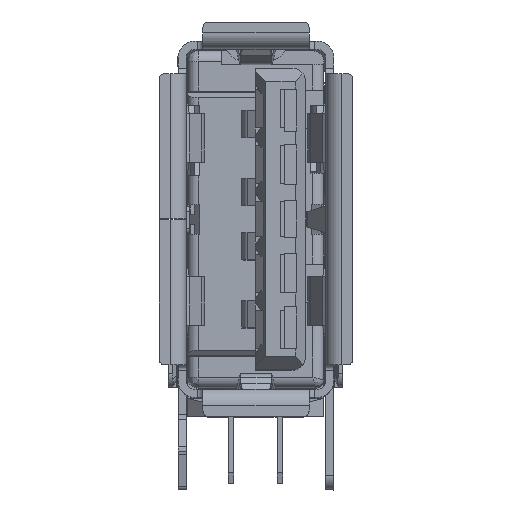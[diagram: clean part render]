
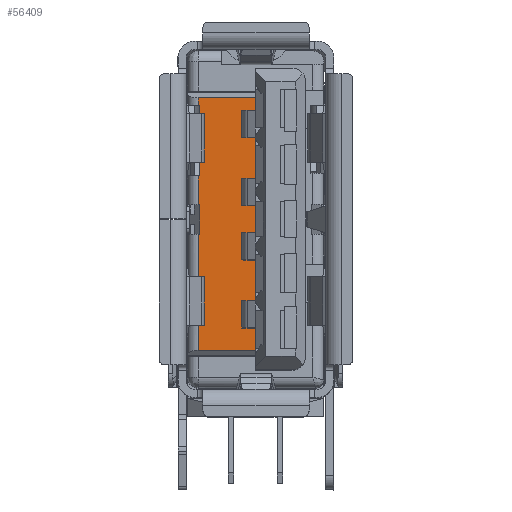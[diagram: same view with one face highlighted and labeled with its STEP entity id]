
A CAD part, top view. The second image highlights one B-rep face of the part: STEP entity #56409.
In plain terms, the highlighted planar face has unit normal (0, 0, 1).
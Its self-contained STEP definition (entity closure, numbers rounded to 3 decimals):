
#46 = ORIENTED_EDGE ( 'NONE', *, *, #74135, .T. ) ;
#1240 = VECTOR ( 'NONE', #19830, 1000. ) ;
#2455 = ORIENTED_EDGE ( 'NONE', *, *, #68808, .T. ) ;
#4025 = VECTOR ( 'NONE', #60709, 1000. ) ;
#4197 = AXIS2_PLACEMENT_3D ( 'NONE', #62936, #84870, #19425 ) ;
#5372 = DIRECTION ( 'NONE',  ( -1., 0., 0. ) ) ;
#6657 = ORIENTED_EDGE ( 'NONE', *, *, #52125, .T. ) ;
#6855 = EDGE_CURVE ( 'NONE', #19934, #87903, #26088, .T. ) ;
#7432 = VECTOR ( 'NONE', #47009, 1000. ) ;
#11514 = VERTEX_POINT ( 'NONE', #66420 ) ;
#12443 = EDGE_CURVE ( 'NONE', #89733, #81826, #86185, .T. ) ;
#12516 = LINE ( 'NONE', #71252, #74132 ) ;
#13197 = FACE_OUTER_BOUND ( 'NONE', #21244, .T. ) ;
#14229 = LINE ( 'NONE', #50551, #50821 ) ;
#14519 = DIRECTION ( 'NONE',  ( -1., 0., 0. ) ) ;
#14822 = ORIENTED_EDGE ( 'NONE', *, *, #34793, .T. ) ;
#16552 = VECTOR ( 'NONE', #48898, 1000. ) ;
#16812 = VERTEX_POINT ( 'NONE', #84341 ) ;
#17603 = DIRECTION ( 'NONE',  ( 1., 0., 0. ) ) ;
#17866 = CARTESIAN_POINT ( 'NONE',  ( -1.055, 0.55, -10.48 ) ) ;
#18363 = EDGE_CURVE ( 'NONE', #81826, #60747, #56077, .T. ) ;
#19425 = DIRECTION ( 'NONE',  ( 0., 1., 0. ) ) ;
#19491 = EDGE_CURVE ( 'NONE', #64188, #16812, #32213, .T. ) ;
#19830 = DIRECTION ( 'NONE',  ( -1., 0., 0. ) ) ;
#19934 = VERTEX_POINT ( 'NONE', #72708 ) ;
#21088 = CARTESIAN_POINT ( 'NONE',  ( -1.055, -0.55, -10.48 ) ) ;
#21215 = CARTESIAN_POINT ( 'NONE',  ( -2.11, -2.76, -10.48 ) ) ;
#21244 = EDGE_LOOP ( 'NONE', ( #75398, #22298, #67837, #65743, #6657, #2455, #46, #76981, #47574, #84046, #71591, #14822, #78786 ) ) ;
#22298 = ORIENTED_EDGE ( 'NONE', *, *, #68637, .T. ) ;
#23085 = VERTEX_POINT ( 'NONE', #64908 ) ;
#24308 = LINE ( 'NONE', #90251, #63141 ) ;
#25056 = EDGE_CURVE ( 'NONE', #87373, #16812, #58937, .T. ) ;
#25169 = VERTEX_POINT ( 'NONE', #89472 ) ;
#26088 = LINE ( 'NONE', #27013, #52079 ) ;
#27013 = CARTESIAN_POINT ( 'NONE',  ( 0., -0.17, -10.48 ) ) ;
#28358 = DIRECTION ( 'NONE',  ( 0., 1., 0. ) ) ;
#32081 = VECTOR ( 'NONE', #14519, 1000. ) ;
#32213 = LINE ( 'NONE', #17866, #7432 ) ;
#34004 = EDGE_CURVE ( 'NONE', #87373, #25169, #42117, .T. ) ;
#34766 = CARTESIAN_POINT ( 'NONE',  ( 0., -4.57, -10.48 ) ) ;
#34793 = EDGE_CURVE ( 'NONE', #25169, #48969, #78554, .T. ) ;
#37415 = VECTOR ( 'NONE', #5372, 1000. ) ;
#41635 = DIRECTION ( 'NONE',  ( 0., 1., 0. ) ) ;
#41705 = CARTESIAN_POINT ( 'NONE',  ( -2.11, -0.17, -10.48 ) ) ;
#42117 = LINE ( 'NONE', #21088, #37415 ) ;
#46652 = CARTESIAN_POINT ( 'NONE',  ( -2.11, 0.55, -10.48 ) ) ;
#47009 = DIRECTION ( 'NONE',  ( 1., 0., 0. ) ) ;
#47437 = VERTEX_POINT ( 'NONE', #54644 ) ;
#47574 = ORIENTED_EDGE ( 'NONE', *, *, #19491, .T. ) ;
#47581 = CARTESIAN_POINT ( 'NONE',  ( 0., 4.47, -10.48 ) ) ;
#48898 = DIRECTION ( 'NONE',  ( 0., -1., 0. ) ) ;
#48969 = VERTEX_POINT ( 'NONE', #73161 ) ;
#48998 = CARTESIAN_POINT ( 'NONE',  ( -2.05, -0.55, -10.48 ) ) ;
#49146 = DIRECTION ( 'NONE',  ( 1., 0., 0. ) ) ;
#50551 = CARTESIAN_POINT ( 'NONE',  ( -2.275, 4.2, -10.48 ) ) ;
#50821 = VECTOR ( 'NONE', #49146, 1000. ) ;
#52079 = VECTOR ( 'NONE', #56175, 1000. ) ;
#52125 = EDGE_CURVE ( 'NONE', #60747, #11514, #14229, .T. ) ;
#54133 = CARTESIAN_POINT ( 'NONE',  ( -2.11, 4.2, -10.48 ) ) ;
#54644 = CARTESIAN_POINT ( 'NONE',  ( -2.04, 1.6, -10.48 ) ) ;
#55238 = VECTOR ( 'NONE', #28358, 1000. ) ;
#56077 = LINE ( 'NONE', #41705, #16552 ) ;
#56175 = DIRECTION ( 'NONE',  ( 0., 1., 0. ) ) ;
#56409 = ADVANCED_FACE ( 'NONE', ( #13197 ), #71479, .T. ) ;
#58025 = CARTESIAN_POINT ( 'NONE',  ( -2.275, 1.6, -10.48 ) ) ;
#58937 = LINE ( 'NONE', #65633, #55238 ) ;
#60709 = DIRECTION ( 'NONE',  ( 0., -1., 0. ) ) ;
#60747 = VERTEX_POINT ( 'NONE', #54133 ) ;
#62936 = CARTESIAN_POINT ( 'NONE',  ( 0.042, -4.996, -10.48 ) ) ;
#63141 = VECTOR ( 'NONE', #17603, 1000. ) ;
#63425 = CARTESIAN_POINT ( 'NONE',  ( -2.04, -0.17, -10.48 ) ) ;
#63801 = DIRECTION ( 'NONE',  ( 0., -1., 0. ) ) ;
#64188 = VERTEX_POINT ( 'NONE', #46652 ) ;
#64908 = CARTESIAN_POINT ( 'NONE',  ( -2.11, 1.6, -10.48 ) ) ;
#65633 = CARTESIAN_POINT ( 'NONE',  ( -2.05, 0., -10.48 ) ) ;
#65655 = CARTESIAN_POINT ( 'NONE',  ( -1.055, 4.47, -10.48 ) ) ;
#65743 = ORIENTED_EDGE ( 'NONE', *, *, #18363, .T. ) ;
#66420 = CARTESIAN_POINT ( 'NONE',  ( -2.04, 4.2, -10.48 ) ) ;
#67837 = ORIENTED_EDGE ( 'NONE', *, *, #12443, .T. ) ;
#68637 = EDGE_CURVE ( 'NONE', #87903, #89733, #12516, .T. ) ;
#68808 = EDGE_CURVE ( 'NONE', #11514, #47437, #93024, .T. ) ;
#68825 = VECTOR ( 'NONE', #78194, 1000. ) ;
#71252 = CARTESIAN_POINT ( 'NONE',  ( 0., -0.17, -10.48 ) ) ;
#71479 = PLANE ( 'NONE',  #4197 ) ;
#71591 = ORIENTED_EDGE ( 'NONE', *, *, #34004, .T. ) ;
#72708 = CARTESIAN_POINT ( 'NONE',  ( 0., -4.81, -10.48 ) ) ;
#73161 = CARTESIAN_POINT ( 'NONE',  ( -2.11, -4.81, -10.48 ) ) ;
#74132 = VECTOR ( 'NONE', #41635, 1000. ) ;
#74135 = EDGE_CURVE ( 'NONE', #47437, #23085, #86189, .T. ) ;
#75398 = ORIENTED_EDGE ( 'NONE', *, *, #6855, .T. ) ;
#76404 = EDGE_CURVE ( 'NONE', #48969, #19934, #24308, .T. ) ;
#76981 = ORIENTED_EDGE ( 'NONE', *, *, #85718, .T. ) ;
#78194 = DIRECTION ( 'NONE',  ( 0., -1., 0. ) ) ;
#78554 = LINE ( 'NONE', #21215, #90941 ) ;
#78786 = ORIENTED_EDGE ( 'NONE', *, *, #76404, .T. ) ;
#81826 = VERTEX_POINT ( 'NONE', #84410 ) ;
#84046 = ORIENTED_EDGE ( 'NONE', *, *, #25056, .F. ) ;
#84341 = CARTESIAN_POINT ( 'NONE',  ( -2.05, 0.55, -10.48 ) ) ;
#84410 = CARTESIAN_POINT ( 'NONE',  ( -2.11, 4.47, -10.48 ) ) ;
#84870 = DIRECTION ( 'NONE',  ( 0., 0., 1. ) ) ;
#85718 = EDGE_CURVE ( 'NONE', #23085, #64188, #93506, .T. ) ;
#85837 = CARTESIAN_POINT ( 'NONE',  ( -2.11, 1.075, -10.48 ) ) ;
#86185 = LINE ( 'NONE', #65655, #1240 ) ;
#86189 = LINE ( 'NONE', #58025, #32081 ) ;
#87373 = VERTEX_POINT ( 'NONE', #48998 ) ;
#87903 = VERTEX_POINT ( 'NONE', #34766 ) ;
#89472 = CARTESIAN_POINT ( 'NONE',  ( -2.11, -0.55, -10.48 ) ) ;
#89733 = VERTEX_POINT ( 'NONE', #47581 ) ;
#90251 = CARTESIAN_POINT ( 'NONE',  ( -1.055, -4.81, -10.48 ) ) ;
#90941 = VECTOR ( 'NONE', #63801, 1000. ) ;
#93024 = LINE ( 'NONE', #63425, #4025 ) ;
#93506 = LINE ( 'NONE', #85837, #68825 ) ;
